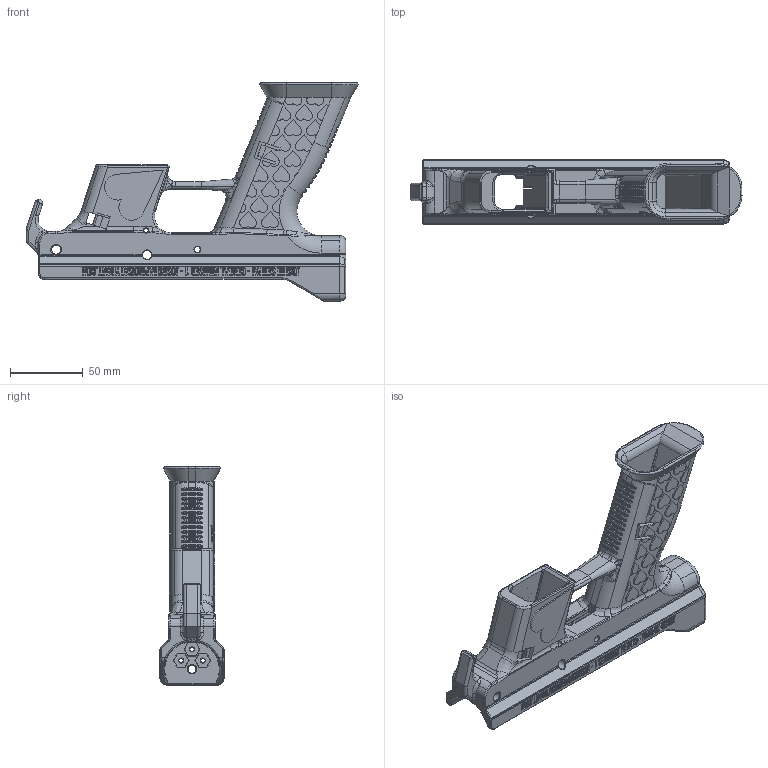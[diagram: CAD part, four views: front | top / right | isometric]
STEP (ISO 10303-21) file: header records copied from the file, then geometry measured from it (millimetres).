
FILE_DESCRIPTION (( 'STEP AP203' ), '1' );
FILE_NAME ('GAB-10_V5_JoshieWoshie9.STEP', '2020-02-07T01:24:33', ( '' ), ( '' ), 'SwSTEP 2.0', 'SolidWorks 2019', '' );
FILE_SCHEMA (( 'CONFIG_CONTROL_DESIGN' ));
Products named in the file (1): GAB-10_V5_JoshieWoshie9
Bounding box: 227.94 x 44 x 149.96 mm (x, y, z)
Volume: 246572.7 mm3; surface area: 89235.1 mm2
Topology: 1 solids, 1 shells, 3584 faces, 9544 edges, 6104 vertices
Faces by surface type: plane 1546, bspline 1268, cylinder 635, torus 83, cone 50, sphere 2
Entity records: 147160 total; most frequent: CARTESIAN_POINT 67965, ORIENTED_EDGE 19032, DIRECTION 11765, EDGE_CURVE 9516, VERTEX_POINT 6104, LINE 5407, VECTOR 5407, EDGE_LOOP 3790
